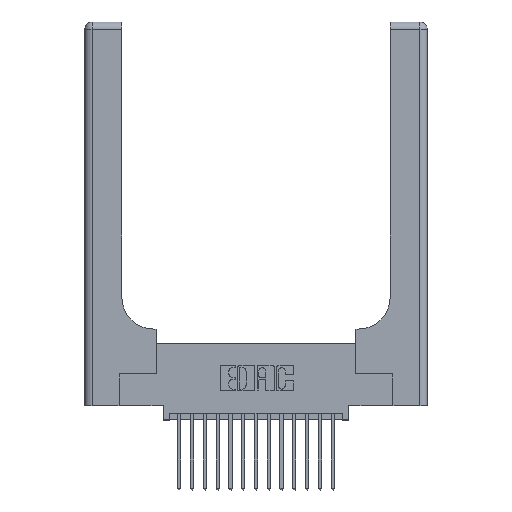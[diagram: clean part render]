
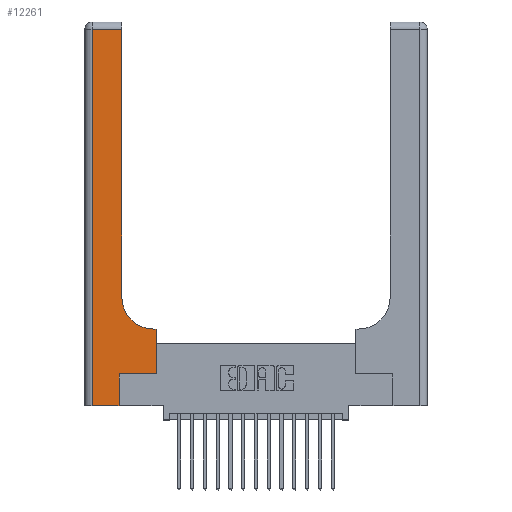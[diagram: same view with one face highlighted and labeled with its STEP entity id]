
A CAD part, top view. The second image highlights one B-rep face of the part: STEP entity #12261.
In plain terms, the highlighted planar face has unit normal (0, 0, 1).
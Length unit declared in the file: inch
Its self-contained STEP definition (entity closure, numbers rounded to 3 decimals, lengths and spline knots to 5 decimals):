
#125 = LINE ( 'NONE', #9945, #15647 ) ;
#1283 = CARTESIAN_POINT ( 'NONE',  ( 0.2915, 2.94, 0.37 ) ) ;
#1593 = DIRECTION ( 'NONE',  ( 0., 1., 0. ) ) ;
#1696 = VERTEX_POINT ( 'NONE', #4074 ) ;
#2019 = EDGE_CURVE ( 'NONE', #2412, #17942, #18940, .T. ) ;
#2126 = VERTEX_POINT ( 'NONE', #7927 ) ;
#2373 = VERTEX_POINT ( 'NONE', #7186 ) ;
#2412 = VERTEX_POINT ( 'NONE', #13116 ) ;
#3030 = EDGE_CURVE ( 'NONE', #16337, #18664, #125, .T. ) ;
#3183 = DIRECTION ( 'NONE',  ( 1., 0., 0. ) ) ;
#3259 = EDGE_CURVE ( 'NONE', #1696, #14080, #13521, .T. ) ;
#3846 = ORIENTED_EDGE ( 'NONE', *, *, #14749, .T. ) ;
#3970 = DIRECTION ( 'NONE',  ( -1., 0., 0. ) ) ;
#4054 = CARTESIAN_POINT ( 'NONE',  ( 0.269, 0.25, 0.37 ) ) ;
#4074 = CARTESIAN_POINT ( 'NONE',  ( 0.5585, 0.25, 0.37 ) ) ;
#4435 = EDGE_LOOP ( 'NONE', ( #8017, #13224, #9356, #10388, #9650, #15024, #5808, #3846, #15241 ) ) ;
#4477 = DIRECTION ( 'NONE',  ( -1., 0., 0. ) ) ;
#4696 = VECTOR ( 'NONE', #5863, 39.37008 ) ;
#4927 = VECTOR ( 'NONE', #3970, 39.37008 ) ;
#5655 = VECTOR ( 'NONE', #14236, 39.37008 ) ;
#5808 = ORIENTED_EDGE ( 'NONE', *, *, #3259, .T. ) ;
#5863 = DIRECTION ( 'NONE',  ( 0., 1., 0. ) ) ;
#6302 = DIRECTION ( 'NONE',  ( -1., 0., 0. ) ) ;
#6438 = CARTESIAN_POINT ( 'NONE',  ( 0.2915, 0.85, 0.37 ) ) ;
#6950 = CARTESIAN_POINT ( 'NONE',  ( 0., 2.94, 0.37 ) ) ;
#6980 = LINE ( 'NONE', #4054, #15956 ) ;
#7018 = LINE ( 'NONE', #10816, #17610 ) ;
#7186 = CARTESIAN_POINT ( 'NONE',  ( 0.06, 2.94, 0.37 ) ) ;
#7927 = CARTESIAN_POINT ( 'NONE',  ( 0.5415, 0.6, 0.37 ) ) ;
#8017 = ORIENTED_EDGE ( 'NONE', *, *, #3030, .T. ) ;
#8168 = DIRECTION ( 'NONE',  ( 0., 0., -1. ) ) ;
#8727 = CARTESIAN_POINT ( 'NONE',  ( 0.269, 0., 0.37 ) ) ;
#9259 = CARTESIAN_POINT ( 'NONE',  ( 0., 0., 0.37 ) ) ;
#9356 = ORIENTED_EDGE ( 'NONE', *, *, #12028, .T. ) ;
#9443 = CARTESIAN_POINT ( 'NONE',  ( 0.5585, 0.6, 0.37 ) ) ;
#9650 = ORIENTED_EDGE ( 'NONE', *, *, #12243, .T. ) ;
#9857 = FACE_OUTER_BOUND ( 'NONE', #4435, .T. ) ;
#9883 = CARTESIAN_POINT ( 'NONE',  ( 0.5415, 0.85, 0.37 ) ) ;
#9945 = CARTESIAN_POINT ( 'NONE',  ( 0.2915, 3., 0.37 ) ) ;
#10089 = LINE ( 'NONE', #15801, #5655 ) ;
#10370 = PLANE ( 'NONE',  #18565 ) ;
#10388 = ORIENTED_EDGE ( 'NONE', *, *, #2019, .T. ) ;
#10567 = LINE ( 'NONE', #8727, #4696 ) ;
#10643 = CARTESIAN_POINT ( 'NONE',  ( 0.5585, 0.25, 0.37 ) ) ;
#10816 = CARTESIAN_POINT ( 'NONE',  ( 0.2915, 0.6, 0.37 ) ) ;
#11123 = VERTEX_POINT ( 'NONE', #13784 ) ;
#12028 = EDGE_CURVE ( 'NONE', #2373, #2412, #10089, .T. ) ;
#12185 = EDGE_CURVE ( 'NONE', #18664, #2373, #18100, .T. ) ;
#12243 = EDGE_CURVE ( 'NONE', #17942, #11123, #10567, .T. ) ;
#12261 = ADVANCED_FACE ( 'NONE', ( #9857 ), #10370, .F. ) ;
#12906 = CARTESIAN_POINT ( 'NONE',  ( 0.269, 0., 0.37 ) ) ;
#13116 = CARTESIAN_POINT ( 'NONE',  ( 0.06, 0., 0.37 ) ) ;
#13224 = ORIENTED_EDGE ( 'NONE', *, *, #12185, .T. ) ;
#13495 = CARTESIAN_POINT ( 'NONE',  ( 0., 3., 0.37 ) ) ;
#13521 = LINE ( 'NONE', #10643, #16080 ) ;
#13784 = CARTESIAN_POINT ( 'NONE',  ( 0.269, 0.25, 0.37 ) ) ;
#14080 = VERTEX_POINT ( 'NONE', #9443 ) ;
#14236 = DIRECTION ( 'NONE',  ( 0., -1., 0. ) ) ;
#14749 = EDGE_CURVE ( 'NONE', #14080, #2126, #7018, .T. ) ;
#15024 = ORIENTED_EDGE ( 'NONE', *, *, #15455, .T. ) ;
#15241 = ORIENTED_EDGE ( 'NONE', *, *, #17915, .T. ) ;
#15455 = EDGE_CURVE ( 'NONE', #11123, #1696, #6980, .T. ) ;
#15647 = VECTOR ( 'NONE', #16246, 39.37008 ) ;
#15801 = CARTESIAN_POINT ( 'NONE',  ( 0.06, 3., 0.37 ) ) ;
#15900 = VECTOR ( 'NONE', #3183, 39.37008 ) ;
#15956 = VECTOR ( 'NONE', #16006, 39.37008 ) ;
#16006 = DIRECTION ( 'NONE',  ( 1., 0., 0. ) ) ;
#16080 = VECTOR ( 'NONE', #1593, 39.37008 ) ;
#16171 = AXIS2_PLACEMENT_3D ( 'NONE', #9883, #8168, #17306 ) ;
#16246 = DIRECTION ( 'NONE',  ( 0., 1., 0. ) ) ;
#16337 = VERTEX_POINT ( 'NONE', #6438 ) ;
#17306 = DIRECTION ( 'NONE',  ( 1., 0., 0. ) ) ;
#17610 = VECTOR ( 'NONE', #6302, 39.37008 ) ;
#17734 = DIRECTION ( 'NONE',  ( 0., 0., -1. ) ) ;
#17915 = EDGE_CURVE ( 'NONE', #2126, #16337, #18700, .T. ) ;
#17942 = VERTEX_POINT ( 'NONE', #12906 ) ;
#18100 = LINE ( 'NONE', #6950, #4927 ) ;
#18565 = AXIS2_PLACEMENT_3D ( 'NONE', #13495, #17734, #4477 ) ;
#18664 = VERTEX_POINT ( 'NONE', #1283 ) ;
#18700 = CIRCLE ( 'NONE', #16171, 0.25 ) ;
#18940 = LINE ( 'NONE', #9259, #15900 ) ;
